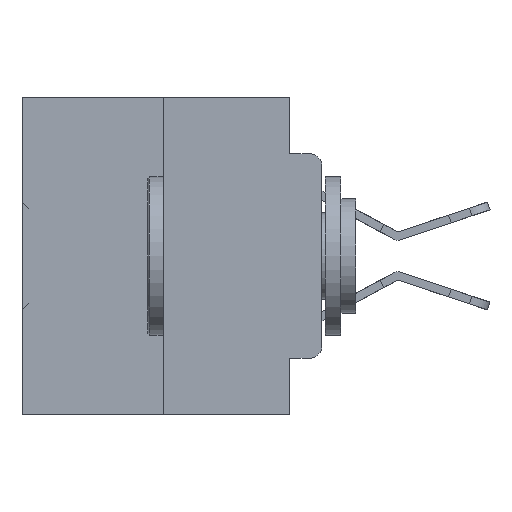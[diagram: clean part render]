
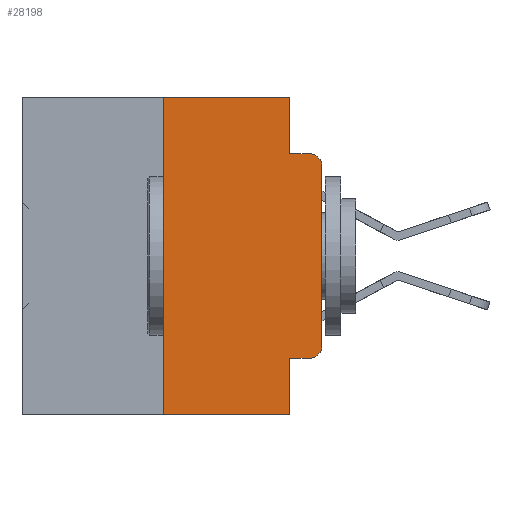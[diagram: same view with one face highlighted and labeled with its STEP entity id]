
A CAD part, left-side view. The second image highlights one B-rep face of the part: STEP entity #28198.
In plain terms, the highlighted planar face has unit normal (-1, 0, 0).
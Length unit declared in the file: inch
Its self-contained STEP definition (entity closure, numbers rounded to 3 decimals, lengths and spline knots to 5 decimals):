
#19 = ORIENTED_EDGE ( 'NONE', *, *, #29017, .F. ) ;
#745 = EDGE_CURVE ( 'NONE', #7716, #28917, #17744, .T. ) ;
#1596 = EDGE_CURVE ( 'NONE', #30082, #38547, #5103, .T. ) ;
#1703 = CARTESIAN_POINT ( 'NONE',  ( 0., 0.473, 0. ) ) ;
#2107 = VERTEX_POINT ( 'NONE', #27924 ) ;
#3828 = CARTESIAN_POINT ( 'NONE',  ( 0., 0., -0.3915 ) ) ;
#4420 = CARTESIAN_POINT ( 'NONE',  ( 0., 0.02, -0.3915 ) ) ;
#4581 = LINE ( 'NONE', #11007, #12433 ) ;
#5103 = LINE ( 'NONE', #17382, #18591 ) ;
#5569 = VERTEX_POINT ( 'NONE', #35582 ) ;
#5970 = CIRCLE ( 'NONE', #37468, 0.02 ) ;
#6686 = CARTESIAN_POINT ( 'NONE',  ( 0., 0.25, 0. ) ) ;
#6955 = VERTEX_POINT ( 'NONE', #28312 ) ;
#7716 = VERTEX_POINT ( 'NONE', #27818 ) ;
#7926 = EDGE_CURVE ( 'NONE', #38547, #28867, #12727, .T. ) ;
#8105 = FACE_OUTER_BOUND ( 'NONE', #23503, .T. ) ;
#9120 = VECTOR ( 'NONE', #12143, 39.37008 ) ;
#10045 = CARTESIAN_POINT ( 'NONE',  ( 0., 0.051, 0. ) ) ;
#10830 = DIRECTION ( 'NONE',  ( 0., 0., -1. ) ) ;
#11007 = CARTESIAN_POINT ( 'NONE',  ( 0., 0.473, -0.5 ) ) ;
#11351 = ORIENTED_EDGE ( 'NONE', *, *, #32893, .F. ) ;
#11392 = LINE ( 'NONE', #24075, #29629 ) ;
#11724 = LINE ( 'NONE', #39113, #9120 ) ;
#12143 = DIRECTION ( 'NONE',  ( 0., -1., 0. ) ) ;
#12433 = VECTOR ( 'NONE', #13440, 39.37008 ) ;
#12727 = LINE ( 'NONE', #15946, #26226 ) ;
#13280 = EDGE_CURVE ( 'NONE', #37955, #7716, #11392, .T. ) ;
#13440 = DIRECTION ( 'NONE',  ( 0., -1., 0. ) ) ;
#14232 = CARTESIAN_POINT ( 'NONE',  ( 0., 0.02, -0.1085 ) ) ;
#15129 = LINE ( 'NONE', #33249, #27420 ) ;
#15344 = ORIENTED_EDGE ( 'NONE', *, *, #16799, .T. ) ;
#15888 = CARTESIAN_POINT ( 'NONE',  ( 0., 0.051, -0.5 ) ) ;
#15946 = CARTESIAN_POINT ( 'NONE',  ( 0., 0.051, 0. ) ) ;
#16000 = AXIS2_PLACEMENT_3D ( 'NONE', #1703, #17373, #38517 ) ;
#16587 = PLANE ( 'NONE',  #16000 ) ;
#16639 = ORIENTED_EDGE ( 'NONE', *, *, #13280, .T. ) ;
#16799 = EDGE_CURVE ( 'NONE', #5569, #22306, #4581, .T. ) ;
#17083 = LINE ( 'NONE', #10045, #26872 ) ;
#17245 = ORIENTED_EDGE ( 'NONE', *, *, #7926, .F. ) ;
#17373 = DIRECTION ( 'NONE',  ( 1., 0., 0. ) ) ;
#17382 = CARTESIAN_POINT ( 'NONE',  ( 0., 0.473, 0. ) ) ;
#17744 = CIRCLE ( 'NONE', #31231, 0.02 ) ;
#18591 = VECTOR ( 'NONE', #29647, 39.37008 ) ;
#20589 = EDGE_CURVE ( 'NONE', #6955, #2107, #5970, .T. ) ;
#21973 = DIRECTION ( 'NONE',  ( 0., 0., -1. ) ) ;
#22306 = VERTEX_POINT ( 'NONE', #15888 ) ;
#22314 = DIRECTION ( 'NONE',  ( 0., 0., -1. ) ) ;
#23130 = DIRECTION ( 'NONE',  ( -1., 0., 0. ) ) ;
#23503 = EDGE_LOOP ( 'NONE', ( #34161, #38982, #11351, #17245, #35175, #37381, #15344, #19, #16639, #38575 ) ) ;
#24075 = CARTESIAN_POINT ( 'NONE',  ( 0., 0.051, -0.4115 ) ) ;
#24371 = CARTESIAN_POINT ( 'NONE',  ( 0., 0.25, 0. ) ) ;
#24955 = CARTESIAN_POINT ( 'NONE',  ( 0., 0.051, -0.0885 ) ) ;
#25000 = DIRECTION ( 'NONE',  ( 0., 0., 1. ) ) ;
#26226 = VECTOR ( 'NONE', #21973, 39.37008 ) ;
#26315 = EDGE_CURVE ( 'NONE', #28917, #6955, #15129, .T. ) ;
#26872 = VECTOR ( 'NONE', #22314, 39.37008 ) ;
#27401 = DIRECTION ( 'NONE',  ( 0., 0., 1. ) ) ;
#27420 = VECTOR ( 'NONE', #27401, 39.37008 ) ;
#27818 = CARTESIAN_POINT ( 'NONE',  ( 0., 0.02, -0.4115 ) ) ;
#27924 = CARTESIAN_POINT ( 'NONE',  ( 0., 0.02, -0.0885 ) ) ;
#28198 = ADVANCED_FACE ( 'NONE', ( #8105 ), #16587, .F. ) ;
#28312 = CARTESIAN_POINT ( 'NONE',  ( 0., 0., -0.1085 ) ) ;
#28867 = VERTEX_POINT ( 'NONE', #24955 ) ;
#28917 = VERTEX_POINT ( 'NONE', #3828 ) ;
#29017 = EDGE_CURVE ( 'NONE', #37955, #22306, #17083, .T. ) ;
#29201 = CARTESIAN_POINT ( 'NONE',  ( 0., 0.051, -0.4115 ) ) ;
#29629 = VECTOR ( 'NONE', #36375, 39.37008 ) ;
#29647 = DIRECTION ( 'NONE',  ( 0., -1., 0. ) ) ;
#30082 = VERTEX_POINT ( 'NONE', #24371 ) ;
#31231 = AXIS2_PLACEMENT_3D ( 'NONE', #4420, #23130, #38616 ) ;
#31743 = EDGE_CURVE ( 'NONE', #5569, #30082, #37085, .T. ) ;
#32893 = EDGE_CURVE ( 'NONE', #28867, #2107, #11724, .T. ) ;
#33249 = CARTESIAN_POINT ( 'NONE',  ( 0., 0., 0. ) ) ;
#33461 = VECTOR ( 'NONE', #25000, 39.37008 ) ;
#34161 = ORIENTED_EDGE ( 'NONE', *, *, #26315, .T. ) ;
#35175 = ORIENTED_EDGE ( 'NONE', *, *, #1596, .F. ) ;
#35196 = DIRECTION ( 'NONE',  ( -1., 0., 0. ) ) ;
#35582 = CARTESIAN_POINT ( 'NONE',  ( 0., 0.25, -0.5 ) ) ;
#36375 = DIRECTION ( 'NONE',  ( 0., -1., 0. ) ) ;
#37085 = LINE ( 'NONE', #6686, #33461 ) ;
#37381 = ORIENTED_EDGE ( 'NONE', *, *, #31743, .F. ) ;
#37468 = AXIS2_PLACEMENT_3D ( 'NONE', #14232, #35196, #10830 ) ;
#37955 = VERTEX_POINT ( 'NONE', #29201 ) ;
#38517 = DIRECTION ( 'NONE',  ( 0., 0., -1. ) ) ;
#38547 = VERTEX_POINT ( 'NONE', #38802 ) ;
#38575 = ORIENTED_EDGE ( 'NONE', *, *, #745, .T. ) ;
#38616 = DIRECTION ( 'NONE',  ( 0., 0., -1. ) ) ;
#38802 = CARTESIAN_POINT ( 'NONE',  ( 0., 0.051, 0. ) ) ;
#38982 = ORIENTED_EDGE ( 'NONE', *, *, #20589, .T. ) ;
#39113 = CARTESIAN_POINT ( 'NONE',  ( 0., 0.051, -0.0885 ) ) ;
